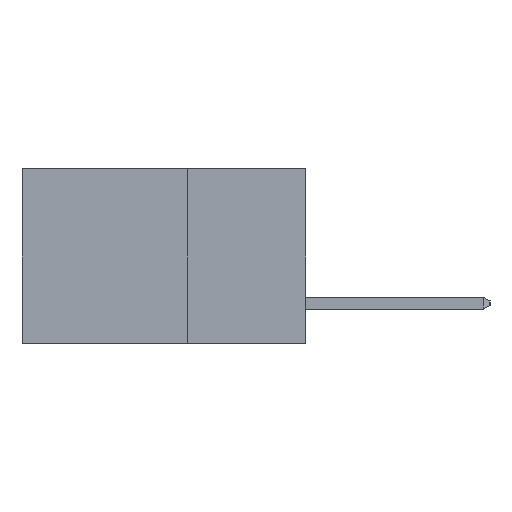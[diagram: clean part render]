
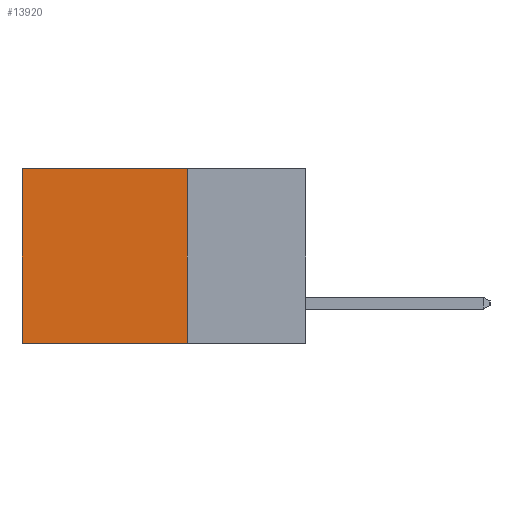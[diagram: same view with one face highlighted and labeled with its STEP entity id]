
A CAD part, left-side view. The second image highlights one B-rep face of the part: STEP entity #13920.
In plain terms, the highlighted planar face has unit normal (-1, 0, 0).
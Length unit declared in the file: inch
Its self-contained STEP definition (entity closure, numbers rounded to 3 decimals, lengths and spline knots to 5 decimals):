
#569 = AXIS2_PLACEMENT_3D ( 'NONE', #3797, #6277, #14784 ) ;
#848 = DIRECTION ( 'NONE',  ( 0., 1., 0. ) ) ;
#1944 = CARTESIAN_POINT ( 'NONE',  ( 0.2615, 0.25, 0. ) ) ;
#2954 = CARTESIAN_POINT ( 'NONE',  ( 0.2615, 0.25, -0.37 ) ) ;
#3797 = CARTESIAN_POINT ( 'NONE',  ( 0.2615, 0.25, -0.37 ) ) ;
#3873 = ORIENTED_EDGE ( 'NONE', *, *, #15232, .T. ) ;
#4746 = ORIENTED_EDGE ( 'NONE', *, *, #11048, .T. ) ;
#4878 = ORIENTED_EDGE ( 'NONE', *, *, #8687, .F. ) ;
#5156 = CARTESIAN_POINT ( 'NONE',  ( 0.2615, 0.25, -0.37 ) ) ;
#5997 = VECTOR ( 'NONE', #12806, 39.37008 ) ;
#6277 = DIRECTION ( 'NONE',  ( 1., 0., 0. ) ) ;
#6426 = ORIENTED_EDGE ( 'NONE', *, *, #9528, .F. ) ;
#6461 = DIRECTION ( 'NONE',  ( 0., 0., -1. ) ) ;
#6520 = LINE ( 'NONE', #8962, #9414 ) ;
#6760 = LINE ( 'NONE', #7014, #9277 ) ;
#7014 = CARTESIAN_POINT ( 'NONE',  ( 0.2615, 0.25, -0.37 ) ) ;
#8589 = VERTEX_POINT ( 'NONE', #13789 ) ;
#8687 = EDGE_CURVE ( 'NONE', #12958, #11691, #15656, .T. ) ;
#8962 = CARTESIAN_POINT ( 'NONE',  ( 0.2615, 0.6, -0.37 ) ) ;
#9277 = VECTOR ( 'NONE', #848, 39.37008 ) ;
#9414 = VECTOR ( 'NONE', #6461, 39.37008 ) ;
#9528 = EDGE_CURVE ( 'NONE', #11691, #8589, #6760, .T. ) ;
#9661 = LINE ( 'NONE', #13695, #15632 ) ;
#10114 = FACE_OUTER_BOUND ( 'NONE', #13198, .T. ) ;
#10134 = VERTEX_POINT ( 'NONE', #13364 ) ;
#11048 = EDGE_CURVE ( 'NONE', #10134, #8589, #6520, .T. ) ;
#11691 = VERTEX_POINT ( 'NONE', #5156 ) ;
#12806 = DIRECTION ( 'NONE',  ( 0., 0., -1. ) ) ;
#12958 = VERTEX_POINT ( 'NONE', #1944 ) ;
#13198 = EDGE_LOOP ( 'NONE', ( #4746, #6426, #4878, #3873 ) ) ;
#13364 = CARTESIAN_POINT ( 'NONE',  ( 0.2615, 0.6, 0. ) ) ;
#13535 = PLANE ( 'NONE',  #569 ) ;
#13695 = CARTESIAN_POINT ( 'NONE',  ( 0.2615, 0.25, 0. ) ) ;
#13748 = DIRECTION ( 'NONE',  ( 0., 1., 0. ) ) ;
#13789 = CARTESIAN_POINT ( 'NONE',  ( 0.2615, 0.6, -0.37 ) ) ;
#13920 = ADVANCED_FACE ( 'NONE', ( #10114 ), #13535, .F. ) ;
#14784 = DIRECTION ( 'NONE',  ( 0., 0., -1. ) ) ;
#15232 = EDGE_CURVE ( 'NONE', #12958, #10134, #9661, .T. ) ;
#15632 = VECTOR ( 'NONE', #13748, 39.37008 ) ;
#15656 = LINE ( 'NONE', #2954, #5997 ) ;
